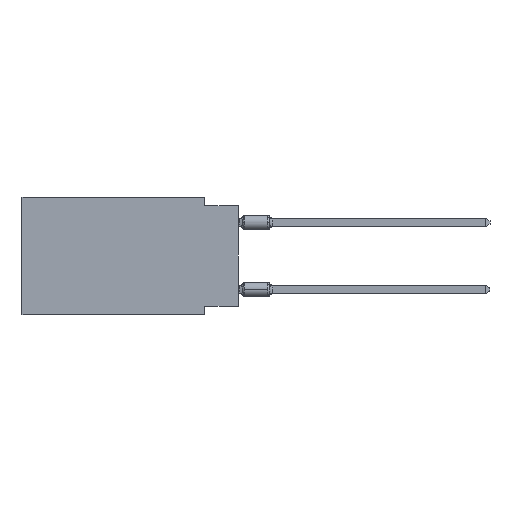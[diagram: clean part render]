
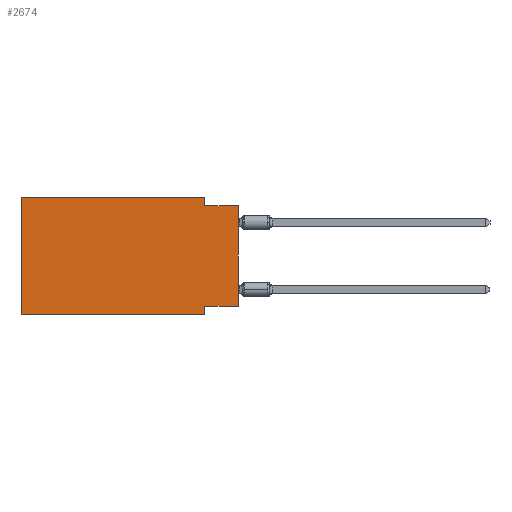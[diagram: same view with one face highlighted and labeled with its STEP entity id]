
A CAD part, left-side view. The second image highlights one B-rep face of the part: STEP entity #2674.
In plain terms, the highlighted planar face has unit normal (-1, 0, 0).
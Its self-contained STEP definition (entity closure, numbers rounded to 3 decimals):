
#1020 = VERTEX_POINT ( 'NONE', #16686 ) ;
#1108 = VECTOR ( 'NONE', #32714, 1000. ) ;
#1319 = LINE ( 'NONE', #11869, #17363 ) ;
#1602 = DIRECTION ( 'NONE',  ( 1., 0., 0. ) ) ;
#1719 = CARTESIAN_POINT ( 'NONE',  ( 0., 16.383, 0. ) ) ;
#1765 = FACE_OUTER_BOUND ( 'NONE', #10259, .T. ) ;
#1851 = VECTOR ( 'NONE', #30963, 1000. ) ;
#2238 = LINE ( 'NONE', #6608, #26715 ) ;
#2397 = VERTEX_POINT ( 'NONE', #29436 ) ;
#2406 = CARTESIAN_POINT ( 'NONE',  ( 0., 0., -0.635 ) ) ;
#2674 = ADVANCED_FACE ( 'NONE', ( #1765 ), #33559, .F. ) ;
#3213 = DIRECTION ( 'NONE',  ( 0., -1., 0. ) ) ;
#4197 = VERTEX_POINT ( 'NONE', #2406 ) ;
#4877 = EDGE_CURVE ( 'NONE', #2397, #32610, #23031, .T. ) ;
#4939 = ORIENTED_EDGE ( 'NONE', *, *, #31615, .F. ) ;
#5408 = EDGE_CURVE ( 'NONE', #28573, #15473, #7254, .T. ) ;
#5815 = CARTESIAN_POINT ( 'NONE',  ( 0., 16.383, 0. ) ) ;
#6608 = CARTESIAN_POINT ( 'NONE',  ( 0., 0., 0. ) ) ;
#6769 = LINE ( 'NONE', #24753, #26541 ) ;
#6964 = DIRECTION ( 'NONE',  ( 0., 0., -1. ) ) ;
#7129 = VERTEX_POINT ( 'NONE', #26404 ) ;
#7254 = LINE ( 'NONE', #1719, #16223 ) ;
#7579 = CARTESIAN_POINT ( 'NONE',  ( 0., 16.383, -8.89 ) ) ;
#7674 = CARTESIAN_POINT ( 'NONE',  ( 0., 2.54, -8.89 ) ) ;
#8591 = EDGE_CURVE ( 'NONE', #7129, #4197, #2238, .T. ) ;
#9052 = EDGE_CURVE ( 'NONE', #32610, #4197, #29141, .T. ) ;
#9275 = DIRECTION ( 'NONE',  ( 0., 0., -1. ) ) ;
#9656 = VECTOR ( 'NONE', #18603, 1000. ) ;
#9695 = ORIENTED_EDGE ( 'NONE', *, *, #4877, .F. ) ;
#10259 = EDGE_LOOP ( 'NONE', ( #16926, #27764, #9695, #4939, #33263, #32193, #26405, #14032 ) ) ;
#11697 = VECTOR ( 'NONE', #3213, 1000. ) ;
#11869 = CARTESIAN_POINT ( 'NONE',  ( 0., 2.54, -8.89 ) ) ;
#12421 = VERTEX_POINT ( 'NONE', #7674 ) ;
#12787 = DIRECTION ( 'NONE',  ( 0., 0., 1. ) ) ;
#14032 = ORIENTED_EDGE ( 'NONE', *, *, #29700, .F. ) ;
#15440 = CARTESIAN_POINT ( 'NONE',  ( 0., 16.383, 0. ) ) ;
#15473 = VERTEX_POINT ( 'NONE', #19002 ) ;
#16223 = VECTOR ( 'NONE', #28343, 1000. ) ;
#16686 = CARTESIAN_POINT ( 'NONE',  ( 0., 2.54, -8.255 ) ) ;
#16926 = ORIENTED_EDGE ( 'NONE', *, *, #8591, .T. ) ;
#17363 = VECTOR ( 'NONE', #9275, 1000. ) ;
#17694 = CARTESIAN_POINT ( 'NONE',  ( 0., 0., -8.255 ) ) ;
#18603 = DIRECTION ( 'NONE',  ( 0., -1., 0. ) ) ;
#19002 = CARTESIAN_POINT ( 'NONE',  ( 0., 16.383, 0. ) ) ;
#20480 = EDGE_CURVE ( 'NONE', #1020, #12421, #1319, .T. ) ;
#22155 = AXIS2_PLACEMENT_3D ( 'NONE', #15440, #1602, #6964 ) ;
#23031 = LINE ( 'NONE', #25967, #1851 ) ;
#24753 = CARTESIAN_POINT ( 'NONE',  ( 0., 16.383, -8.89 ) ) ;
#25313 = LINE ( 'NONE', #17694, #1108 ) ;
#25896 = CARTESIAN_POINT ( 'NONE',  ( 0., 2.54, -0.635 ) ) ;
#25967 = CARTESIAN_POINT ( 'NONE',  ( 0., 2.54, 0. ) ) ;
#26404 = CARTESIAN_POINT ( 'NONE',  ( 0., 0., -8.255 ) ) ;
#26405 = ORIENTED_EDGE ( 'NONE', *, *, #20480, .F. ) ;
#26541 = VECTOR ( 'NONE', #32670, 1000. ) ;
#26715 = VECTOR ( 'NONE', #12787, 1000. ) ;
#26722 = CARTESIAN_POINT ( 'NONE',  ( 0., 0., -0.635 ) ) ;
#27764 = ORIENTED_EDGE ( 'NONE', *, *, #9052, .F. ) ;
#28343 = DIRECTION ( 'NONE',  ( 0., 0., 1. ) ) ;
#28573 = VERTEX_POINT ( 'NONE', #7579 ) ;
#29141 = LINE ( 'NONE', #26722, #9656 ) ;
#29436 = CARTESIAN_POINT ( 'NONE',  ( 0., 2.54, 0. ) ) ;
#29478 = LINE ( 'NONE', #5815, #11697 ) ;
#29700 = EDGE_CURVE ( 'NONE', #7129, #1020, #25313, .T. ) ;
#30035 = EDGE_CURVE ( 'NONE', #28573, #12421, #6769, .T. ) ;
#30963 = DIRECTION ( 'NONE',  ( 0., 0., -1. ) ) ;
#31615 = EDGE_CURVE ( 'NONE', #15473, #2397, #29478, .T. ) ;
#32193 = ORIENTED_EDGE ( 'NONE', *, *, #30035, .T. ) ;
#32610 = VERTEX_POINT ( 'NONE', #25896 ) ;
#32670 = DIRECTION ( 'NONE',  ( 0., -1., 0. ) ) ;
#32714 = DIRECTION ( 'NONE',  ( 0., 1., 0. ) ) ;
#33263 = ORIENTED_EDGE ( 'NONE', *, *, #5408, .F. ) ;
#33559 = PLANE ( 'NONE',  #22155 ) ;
